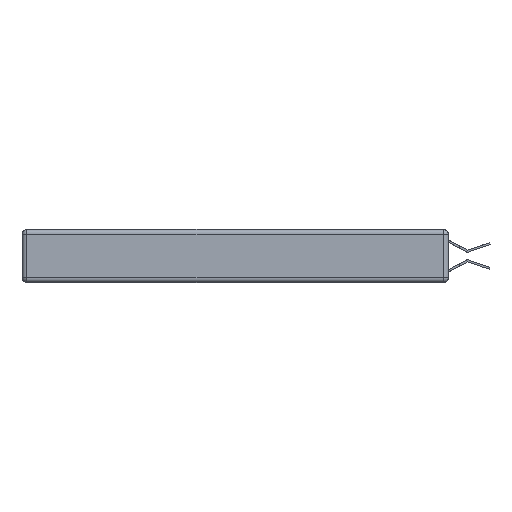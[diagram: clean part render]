
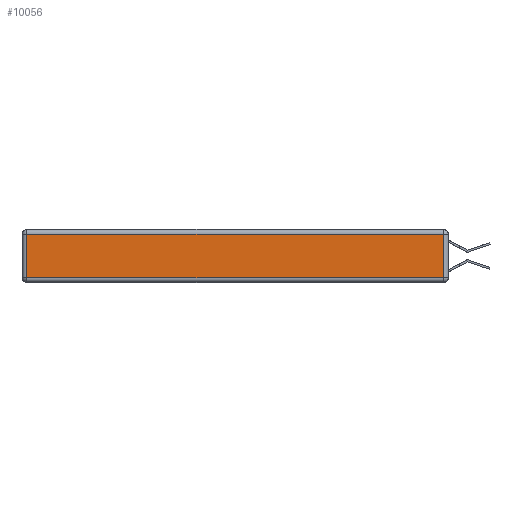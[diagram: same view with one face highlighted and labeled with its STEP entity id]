
A CAD part, left-side view. The second image highlights one B-rep face of the part: STEP entity #10056.
In plain terms, the highlighted planar face has unit normal (-1, 0, 0).
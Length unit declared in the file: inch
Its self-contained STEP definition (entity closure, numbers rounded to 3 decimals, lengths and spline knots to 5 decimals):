
#628 = DIRECTION ( 'NONE',  ( 0., 0., 1. ) ) ;
#678 = AXIS2_PLACEMENT_3D ( 'NONE', #22207, #17170, #6223 ) ;
#778 = ORIENTED_EDGE ( 'NONE', *, *, #20232, .T. ) ;
#1829 = CARTESIAN_POINT ( 'NONE',  ( 0., 2.72, -0.343 ) ) ;
#1879 = LINE ( 'NONE', #9251, #11275 ) ;
#2650 = CARTESIAN_POINT ( 'NONE',  ( 0., 0., -0.313 ) ) ;
#3503 = EDGE_CURVE ( 'NONE', #10770, #11271, #12226, .T. ) ;
#4470 = FACE_OUTER_BOUND ( 'NONE', #20289, .T. ) ;
#6223 = DIRECTION ( 'NONE',  ( 0., 0., 1. ) ) ;
#6487 = VECTOR ( 'NONE', #12118, 39.37008 ) ;
#7977 = CARTESIAN_POINT ( 'NONE',  ( 0., 2.72, -0.313 ) ) ;
#9050 = ORIENTED_EDGE ( 'NONE', *, *, #12699, .T. ) ;
#9251 = CARTESIAN_POINT ( 'NONE',  ( 0., 2.75, -0.03 ) ) ;
#9451 = CARTESIAN_POINT ( 'NONE',  ( 0., 2.72, -0.03 ) ) ;
#9774 = DIRECTION ( 'NONE',  ( 0., -1., 0. ) ) ;
#9807 = CARTESIAN_POINT ( 'NONE',  ( 0., 0.03, -0.313 ) ) ;
#9960 = PLANE ( 'NONE',  #678 ) ;
#10056 = ADVANCED_FACE ( 'NONE', ( #4470 ), #9960, .T. ) ;
#10770 = VERTEX_POINT ( 'NONE', #9451 ) ;
#11271 = VERTEX_POINT ( 'NONE', #7977 ) ;
#11275 = VECTOR ( 'NONE', #21483, 39.37008 ) ;
#11817 = VERTEX_POINT ( 'NONE', #9807 ) ;
#12118 = DIRECTION ( 'NONE',  ( 0., 0., -1. ) ) ;
#12226 = LINE ( 'NONE', #1829, #6487 ) ;
#12699 = EDGE_CURVE ( 'NONE', #11817, #16166, #16622, .T. ) ;
#14501 = VECTOR ( 'NONE', #628, 39.37008 ) ;
#14859 = CARTESIAN_POINT ( 'NONE',  ( 0., 0.03, -0.343 ) ) ;
#14914 = ORIENTED_EDGE ( 'NONE', *, *, #3503, .T. ) ;
#15095 = ORIENTED_EDGE ( 'NONE', *, *, #16923, .T. ) ;
#16166 = VERTEX_POINT ( 'NONE', #17504 ) ;
#16622 = LINE ( 'NONE', #14859, #14501 ) ;
#16923 = EDGE_CURVE ( 'NONE', #16166, #10770, #1879, .T. ) ;
#17170 = DIRECTION ( 'NONE',  ( -1., 0., 0. ) ) ;
#17504 = CARTESIAN_POINT ( 'NONE',  ( 0., 0.03, -0.03 ) ) ;
#19573 = VECTOR ( 'NONE', #9774, 39.37008 ) ;
#20232 = EDGE_CURVE ( 'NONE', #11271, #11817, #22012, .T. ) ;
#20289 = EDGE_LOOP ( 'NONE', ( #778, #9050, #15095, #14914 ) ) ;
#21483 = DIRECTION ( 'NONE',  ( 0., 1., 0. ) ) ;
#22012 = LINE ( 'NONE', #2650, #19573 ) ;
#22207 = CARTESIAN_POINT ( 'NONE',  ( 0., 0., -0.343 ) ) ;
